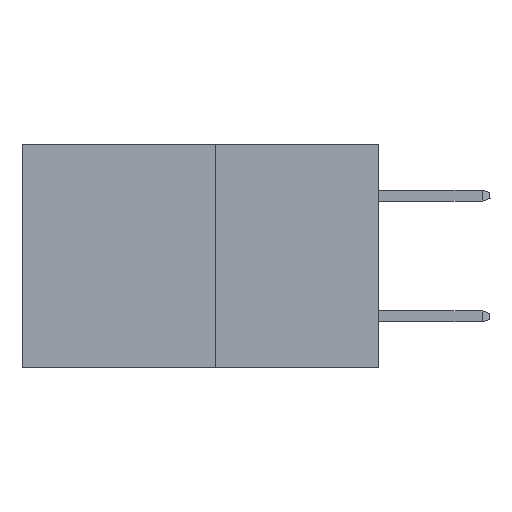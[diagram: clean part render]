
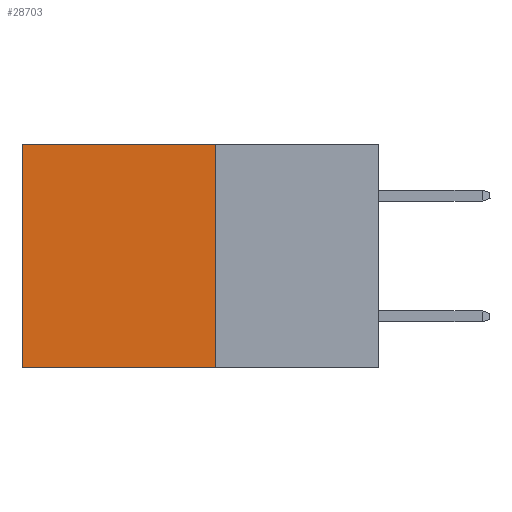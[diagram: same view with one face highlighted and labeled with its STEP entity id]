
A CAD part, left-side view. The second image highlights one B-rep face of the part: STEP entity #28703.
In plain terms, the highlighted planar face has unit normal (-1, 0, 0).
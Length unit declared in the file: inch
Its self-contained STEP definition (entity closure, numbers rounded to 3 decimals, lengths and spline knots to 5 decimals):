
#709 = DIRECTION ( 'NONE',  ( 1., 0., 0. ) ) ;
#2414 = DIRECTION ( 'NONE',  ( 0., 0., -1. ) ) ;
#3527 = CARTESIAN_POINT ( 'NONE',  ( 0.277, 0.27, 0. ) ) ;
#3858 = EDGE_LOOP ( 'NONE', ( #32552, #18597, #8253, #9865 ) ) ;
#4451 = CARTESIAN_POINT ( 'NONE',  ( 0.277, 0.27, 0. ) ) ;
#6990 = VERTEX_POINT ( 'NONE', #4451 ) ;
#8253 = ORIENTED_EDGE ( 'NONE', *, *, #22645, .F. ) ;
#8306 = DIRECTION ( 'NONE',  ( 0., 1., 0. ) ) ;
#9571 = VECTOR ( 'NONE', #2414, 39.37008 ) ;
#9865 = ORIENTED_EDGE ( 'NONE', *, *, #24247, .T. ) ;
#10191 = FACE_OUTER_BOUND ( 'NONE', #3858, .T. ) ;
#10227 = CARTESIAN_POINT ( 'NONE',  ( 0.277, 0.27, -0.37 ) ) ;
#15696 = VECTOR ( 'NONE', #16606, 39.37008 ) ;
#15749 = CARTESIAN_POINT ( 'NONE',  ( 0.277, 0.59, -0.37 ) ) ;
#16235 = EDGE_CURVE ( 'NONE', #30118, #16420, #24735, .T. ) ;
#16406 = PLANE ( 'NONE',  #29608 ) ;
#16420 = VERTEX_POINT ( 'NONE', #32508 ) ;
#16546 = LINE ( 'NONE', #10227, #9571 ) ;
#16606 = DIRECTION ( 'NONE',  ( 0., 1., 0. ) ) ;
#16786 = CARTESIAN_POINT ( 'NONE',  ( 0.277, 0.27, -0.37 ) ) ;
#18225 = DIRECTION ( 'NONE',  ( 0., 0., -1. ) ) ;
#18597 = ORIENTED_EDGE ( 'NONE', *, *, #16235, .F. ) ;
#18997 = DIRECTION ( 'NONE',  ( 0., 0., -1. ) ) ;
#19615 = LINE ( 'NONE', #15749, #27418 ) ;
#22635 = LINE ( 'NONE', #3527, #15696 ) ;
#22645 = EDGE_CURVE ( 'NONE', #6990, #30118, #16546, .T. ) ;
#23987 = CARTESIAN_POINT ( 'NONE',  ( 0.277, 0.27, -0.37 ) ) ;
#24247 = EDGE_CURVE ( 'NONE', #6990, #30422, #22635, .T. ) ;
#24735 = LINE ( 'NONE', #23987, #26370 ) ;
#26370 = VECTOR ( 'NONE', #8306, 39.37008 ) ;
#27418 = VECTOR ( 'NONE', #18225, 39.37008 ) ;
#28540 = EDGE_CURVE ( 'NONE', #30422, #16420, #19615, .T. ) ;
#28703 = ADVANCED_FACE ( 'NONE', ( #10191 ), #16406, .F. ) ;
#29608 = AXIS2_PLACEMENT_3D ( 'NONE', #32026, #709, #18997 ) ;
#30118 = VERTEX_POINT ( 'NONE', #16786 ) ;
#30422 = VERTEX_POINT ( 'NONE', #31451 ) ;
#31451 = CARTESIAN_POINT ( 'NONE',  ( 0.277, 0.59, 0. ) ) ;
#32026 = CARTESIAN_POINT ( 'NONE',  ( 0.277, 0.27, -0.37 ) ) ;
#32508 = CARTESIAN_POINT ( 'NONE',  ( 0.277, 0.59, -0.37 ) ) ;
#32552 = ORIENTED_EDGE ( 'NONE', *, *, #28540, .T. ) ;
